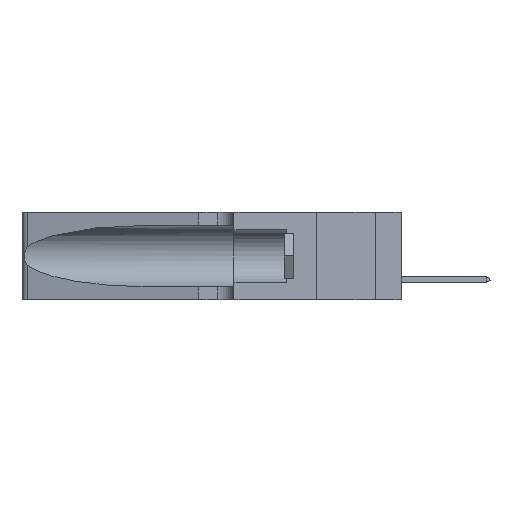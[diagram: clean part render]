
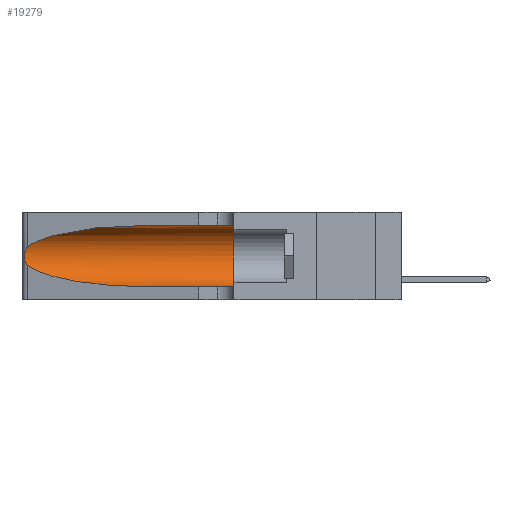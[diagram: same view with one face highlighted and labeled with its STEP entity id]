
A CAD part, left-side view. The second image highlights one B-rep face of the part: STEP entity #19279.
In plain terms, the highlighted cylindrical face has radius 3.308 mm (diameter 6.617 mm), a partial arc.
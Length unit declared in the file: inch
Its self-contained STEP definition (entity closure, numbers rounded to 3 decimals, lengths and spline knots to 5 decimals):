
#159 = CARTESIAN_POINT ( 'NONE',  ( 0.25789, 1.23486, 0.15765 ) ) ;
#287 = CARTESIAN_POINT ( 'NONE',  ( 0.25639, 1.23186, 0.15144 ) ) ;
#854 = CARTESIAN_POINT ( 'NONE',  ( 0.25487, 1.22718, 0.14631 ) ) ;
#1279 = CARTESIAN_POINT ( 'NONE',  ( 0.1305, 0.72297, 0.05475 ) ) ;
#1709 = CARTESIAN_POINT ( 'NONE',  ( 0.1305, 0.72297, 0.05475 ) ) ;
#2187 = DIRECTION ( 'NONE',  ( 0., 0., -1. ) ) ;
#2498 =( BOUNDED_CURVE ( )  B_SPLINE_CURVE ( 3, ( #36527, #5474, #39672, #33470 ),
 .UNSPECIFIED., .F., .T. ) 
 B_SPLINE_CURVE_WITH_KNOTS ( ( 4, 4 ),
 ( 1.5708, 2.84003 ),
 .UNSPECIFIED. ) 
 CURVE ( )  GEOMETRIC_REPRESENTATION_ITEM ( )  RATIONAL_B_SPLINE_CURVE ( ( 1., 0.87, 0.87, 1. ) ) 
 REPRESENTATION_ITEM ( '' )  );
#3745 = CARTESIAN_POINT ( 'NONE',  ( 0.25555, 1.22993, 0.14849 ) ) ;
#4753 = CARTESIAN_POINT ( 'NONE',  ( 0.18966, 0.96281, 0.05475 ) ) ;
#5474 = CARTESIAN_POINT ( 'NONE',  ( 0.18966, 0.96281, 0.31525 ) ) ;
#5610 = LINE ( 'NONE', #37230, #38058 ) ;
#5985 = VECTOR ( 'NONE', #36825, 39.37008 ) ;
#6794 = CARTESIAN_POINT ( 'NONE',  ( 0.26075, 1.23896, 0.19203 ) ) ;
#7767 = CARTESIAN_POINT ( 'NONE',  ( 0.2373, 1.15595, 0.08982 ) ) ;
#9643 = CARTESIAN_POINT ( 'NONE',  ( 0.25487, 1.22718, 0.22369 ) ) ;
#10069 = CARTESIAN_POINT ( 'NONE',  ( 0.26018, 1.23835, 0.19895 ) ) ;
#11008 = CARTESIAN_POINT ( 'NONE',  ( 0.1305, 1.61858, 0.185 ) ) ;
#11305 = B_SPLINE_CURVE_WITH_KNOTS ( 'NONE', 3,
 ( #18416, #27616, #40243, #21473, #13085, #10069, #6794, #35237, #22743, #16374, #159, #287, #3745, #19403 ),
 .UNSPECIFIED., .F., .F.,
 ( 4, 2, 2, 2, 2, 2, 4 ),
 ( 0., 0.00027, 0.00053, 0.00107, 0.0016, 0.00187, 0.00214 ),
 .UNSPECIFIED. ) ;
#12517 = AXIS2_PLACEMENT_3D ( 'NONE', #11008, #32961, #2187 ) ;
#13085 = CARTESIAN_POINT ( 'NONE',  ( 0.25854, 1.2359, 0.20912 ) ) ;
#14232 = VERTEX_POINT ( 'NONE', #17833 ) ;
#14371 = EDGE_CURVE ( 'NONE', #14232, #27489, #18626, .T. ) ;
#14661 = CARTESIAN_POINT ( 'NONE',  ( 0.1305, 0.35, 0.185 ) ) ;
#14980 = EDGE_CURVE ( 'NONE', #30123, #17097, #40369, .T. ) ;
#15211 = CARTESIAN_POINT ( 'NONE',  ( 0.1305, 1.61858, 0.31525 ) ) ;
#16321 = EDGE_LOOP ( 'NONE', ( #28630, #32331, #40516, #40658, #36479, #18038 ) ) ;
#16343 = EDGE_CURVE ( 'NONE', #27489, #20609, #5610, .T. ) ;
#16374 = CARTESIAN_POINT ( 'NONE',  ( 0.25856, 1.23593, 0.16098 ) ) ;
#17097 = VERTEX_POINT ( 'NONE', #30319 ) ;
#17833 = CARTESIAN_POINT ( 'NONE',  ( 0.25487, 1.22718, 0.14631 ) ) ;
#18038 = ORIENTED_EDGE ( 'NONE', *, *, #14980, .F. ) ;
#18416 = CARTESIAN_POINT ( 'NONE',  ( 0.25487, 1.22718, 0.22369 ) ) ;
#18626 =( BOUNDED_CURVE ( )  B_SPLINE_CURVE ( 3, ( #854, #7767, #4753, #1709 ),
 .UNSPECIFIED., .F., .T. ) 
 B_SPLINE_CURVE_WITH_KNOTS ( ( 4, 4 ),
 ( 3.44316, 4.71239 ),
 .UNSPECIFIED. ) 
 CURVE ( )  GEOMETRIC_REPRESENTATION_ITEM ( )  RATIONAL_B_SPLINE_CURVE ( ( 1., 0.87, 0.87, 1. ) ) 
 REPRESENTATION_ITEM ( '' )  );
#19279 = ADVANCED_FACE ( 'NONE', ( #32587 ), #23292, .F. ) ;
#19403 = CARTESIAN_POINT ( 'NONE',  ( 0.25487, 1.22718, 0.14631 ) ) ;
#20609 = VERTEX_POINT ( 'NONE', #40692 ) ;
#21473 = CARTESIAN_POINT ( 'NONE',  ( 0.25787, 1.23484, 0.2124 ) ) ;
#22540 = VERTEX_POINT ( 'NONE', #9643 ) ;
#22743 = CARTESIAN_POINT ( 'NONE',  ( 0.26017, 1.23833, 0.17102 ) ) ;
#22980 = CARTESIAN_POINT ( 'NONE',  ( 0.1305, 0.72297, 0.31525 ) ) ;
#23292 = CYLINDRICAL_SURFACE ( 'NONE', #12517, 0.13025 ) ;
#27456 = DIRECTION ( 'NONE',  ( 0., 1., 0. ) ) ;
#27489 = VERTEX_POINT ( 'NONE', #1279 ) ;
#27612 = EDGE_CURVE ( 'NONE', #30123, #22540, #2498, .T. ) ;
#27616 = CARTESIAN_POINT ( 'NONE',  ( 0.25555, 1.22994, 0.2215 ) ) ;
#28630 = ORIENTED_EDGE ( 'NONE', *, *, #27612, .T. ) ;
#29029 = AXIS2_PLACEMENT_3D ( 'NONE', #14661, #27456, #36684 ) ;
#30123 = VERTEX_POINT ( 'NONE', #22980 ) ;
#30319 = CARTESIAN_POINT ( 'NONE',  ( 0.1305, 0.35, 0.31525 ) ) ;
#32331 = ORIENTED_EDGE ( 'NONE', *, *, #36771, .T. ) ;
#32587 = FACE_OUTER_BOUND ( 'NONE', #16321, .T. ) ;
#32961 = DIRECTION ( 'NONE',  ( 0., -1., 0. ) ) ;
#33470 = CARTESIAN_POINT ( 'NONE',  ( 0.25487, 1.22718, 0.22369 ) ) ;
#33870 = DIRECTION ( 'NONE',  ( 0., -1., 0. ) ) ;
#33909 = CIRCLE ( 'NONE', #29029, 0.13025 ) ;
#35237 = CARTESIAN_POINT ( 'NONE',  ( 0.26075, 1.23896, 0.178 ) ) ;
#35341 = EDGE_CURVE ( 'NONE', #17097, #20609, #33909, .T. ) ;
#36479 = ORIENTED_EDGE ( 'NONE', *, *, #35341, .F. ) ;
#36527 = CARTESIAN_POINT ( 'NONE',  ( 0.1305, 0.72297, 0.31525 ) ) ;
#36684 = DIRECTION ( 'NONE',  ( 0., 0., 1. ) ) ;
#36771 = EDGE_CURVE ( 'NONE', #22540, #14232, #11305, .T. ) ;
#36825 = DIRECTION ( 'NONE',  ( 0., -1., 0. ) ) ;
#37230 = CARTESIAN_POINT ( 'NONE',  ( 0.1305, 1.61858, 0.05475 ) ) ;
#38058 = VECTOR ( 'NONE', #33870, 39.37008 ) ;
#39672 = CARTESIAN_POINT ( 'NONE',  ( 0.2373, 1.15595, 0.28018 ) ) ;
#40243 = CARTESIAN_POINT ( 'NONE',  ( 0.25639, 1.23184, 0.21858 ) ) ;
#40369 = LINE ( 'NONE', #15211, #5985 ) ;
#40516 = ORIENTED_EDGE ( 'NONE', *, *, #14371, .T. ) ;
#40658 = ORIENTED_EDGE ( 'NONE', *, *, #16343, .T. ) ;
#40692 = CARTESIAN_POINT ( 'NONE',  ( 0.1305, 0.35, 0.05475 ) ) ;
